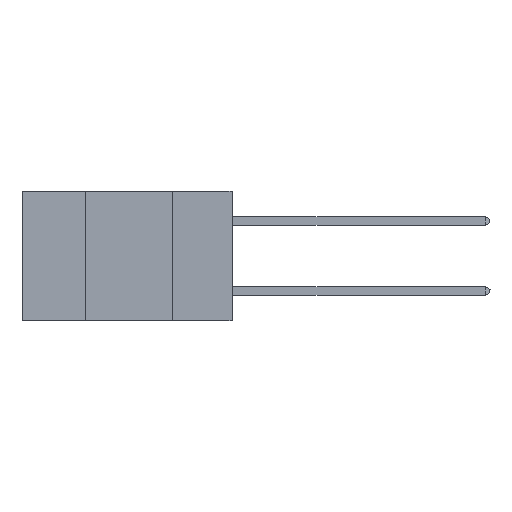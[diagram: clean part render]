
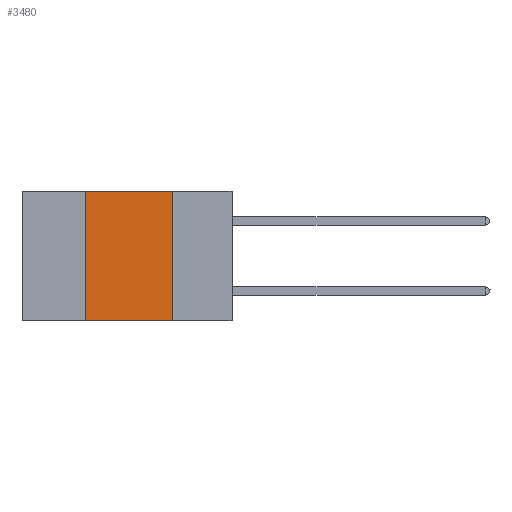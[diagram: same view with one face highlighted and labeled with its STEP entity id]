
A CAD part, left-side view. The second image highlights one B-rep face of the part: STEP entity #3480.
In plain terms, the highlighted planar face has unit normal (-1, 0, 0).
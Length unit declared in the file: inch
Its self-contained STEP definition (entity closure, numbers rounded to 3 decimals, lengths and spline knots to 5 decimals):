
#246 = AXIS2_PLACEMENT_3D ( 'NONE', #23907, #24066, #10666 ) ;
#3480 = ADVANCED_FACE ( 'NONE', ( #23387 ), #22016, .F. ) ;
#3660 = EDGE_CURVE ( 'NONE', #18533, #10184, #11144, .T. ) ;
#4487 = VECTOR ( 'NONE', #5037, 39.37008 ) ;
#4700 = CARTESIAN_POINT ( 'NONE',  ( 0., 0.42, 0. ) ) ;
#5037 = DIRECTION ( 'NONE',  ( 0., -1., 0. ) ) ;
#5311 = DIRECTION ( 'NONE',  ( 0., -1., 0. ) ) ;
#5589 = CARTESIAN_POINT ( 'NONE',  ( 0., 0.17, 0. ) ) ;
#6547 = VERTEX_POINT ( 'NONE', #5589 ) ;
#6814 = DIRECTION ( 'NONE',  ( 0., 0., -1. ) ) ;
#6897 = CARTESIAN_POINT ( 'NONE',  ( 0., 0.17, 0. ) ) ;
#7484 = EDGE_CURVE ( 'NONE', #18533, #12654, #20793, .T. ) ;
#8908 = CARTESIAN_POINT ( 'NONE',  ( 0., 0.6, -0.37 ) ) ;
#9579 = ORIENTED_EDGE ( 'NONE', *, *, #7484, .F. ) ;
#9587 = LINE ( 'NONE', #16717, #4487 ) ;
#10184 = VERTEX_POINT ( 'NONE', #11465 ) ;
#10666 = DIRECTION ( 'NONE',  ( 0., 0., -1. ) ) ;
#10876 = ORIENTED_EDGE ( 'NONE', *, *, #3660, .T. ) ;
#11101 = CARTESIAN_POINT ( 'NONE',  ( 0., 0.42, -0.37 ) ) ;
#11144 = LINE ( 'NONE', #8908, #16233 ) ;
#11465 = CARTESIAN_POINT ( 'NONE',  ( 0., 0.17, -0.37 ) ) ;
#12382 = DIRECTION ( 'NONE',  ( 0., 0., 1. ) ) ;
#12654 = VERTEX_POINT ( 'NONE', #13569 ) ;
#12985 = EDGE_CURVE ( 'NONE', #12654, #6547, #9587, .T. ) ;
#13472 = LINE ( 'NONE', #6897, #20026 ) ;
#13569 = CARTESIAN_POINT ( 'NONE',  ( 0., 0.42, 0. ) ) ;
#14255 = VECTOR ( 'NONE', #12382, 39.37008 ) ;
#16233 = VECTOR ( 'NONE', #5311, 39.37008 ) ;
#16717 = CARTESIAN_POINT ( 'NONE',  ( 0., 0.6, 0. ) ) ;
#17008 = ORIENTED_EDGE ( 'NONE', *, *, #12985, .F. ) ;
#18533 = VERTEX_POINT ( 'NONE', #11101 ) ;
#20026 = VECTOR ( 'NONE', #6814, 39.37008 ) ;
#20793 = LINE ( 'NONE', #4700, #14255 ) ;
#22016 = PLANE ( 'NONE',  #246 ) ;
#22422 = ORIENTED_EDGE ( 'NONE', *, *, #23457, .F. ) ;
#23046 = EDGE_LOOP ( 'NONE', ( #22422, #17008, #9579, #10876 ) ) ;
#23387 = FACE_OUTER_BOUND ( 'NONE', #23046, .T. ) ;
#23457 = EDGE_CURVE ( 'NONE', #6547, #10184, #13472, .T. ) ;
#23907 = CARTESIAN_POINT ( 'NONE',  ( 0., 0.6, 0. ) ) ;
#24066 = DIRECTION ( 'NONE',  ( 1., 0., 0. ) ) ;
